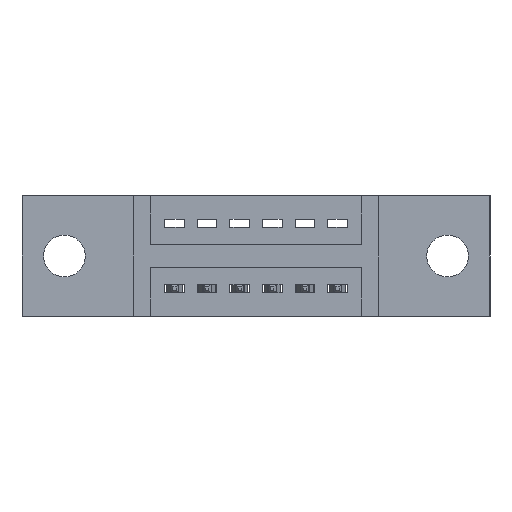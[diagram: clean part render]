
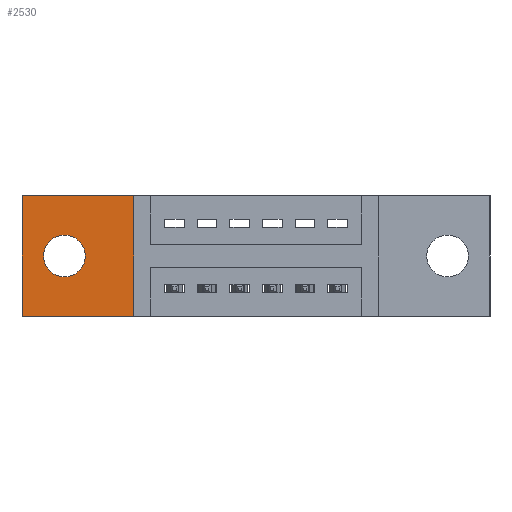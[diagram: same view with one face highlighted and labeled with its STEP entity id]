
A CAD part, front view. The second image highlights one B-rep face of the part: STEP entity #2530.
In plain terms, the highlighted planar face has unit normal (0, -1, 0).
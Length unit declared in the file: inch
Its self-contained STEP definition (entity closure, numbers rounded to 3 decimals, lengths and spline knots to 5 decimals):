
#359 = CARTESIAN_POINT ( 'NONE',  ( 0.3425, 0.11, 0. ) ) ;
#462 = CARTESIAN_POINT ( 'NONE',  ( 0., 0.11, 0. ) ) ;
#1074 = VERTEX_POINT ( 'NONE', #7972 ) ;
#1160 = DIRECTION ( 'NONE',  ( 0., 0., -1. ) ) ;
#1195 = EDGE_CURVE ( 'NONE', #3019, #8788, #3994, .T. ) ;
#1220 = FACE_OUTER_BOUND ( 'NONE', #4221, .T. ) ;
#1246 = CARTESIAN_POINT ( 'NONE',  ( 0., 0.11, 0. ) ) ;
#1267 = EDGE_CURVE ( 'NONE', #8788, #7322, #4454, .T. ) ;
#1342 = AXIS2_PLACEMENT_3D ( 'NONE', #3920, #8228, #3813 ) ;
#1652 = ORIENTED_EDGE ( 'NONE', *, *, #5545, .T. ) ;
#1711 = CARTESIAN_POINT ( 'NONE',  ( 0.3425, 0.11, -0.37 ) ) ;
#1998 = VERTEX_POINT ( 'NONE', #4683 ) ;
#2013 = DIRECTION ( 'NONE',  ( -1., 0., 0. ) ) ;
#2136 = CARTESIAN_POINT ( 'NONE',  ( 0.3425, 0.11, 0. ) ) ;
#2402 = ORIENTED_EDGE ( 'NONE', *, *, #1267, .T. ) ;
#2413 = PLANE ( 'NONE',  #1342 ) ;
#2455 = VECTOR ( 'NONE', #8873, 39.37008 ) ;
#2530 = ADVANCED_FACE ( 'NONE', ( #9464, #1220 ), #2413, .T. ) ;
#2647 = VECTOR ( 'NONE', #2013, 39.37008 ) ;
#2788 = ORIENTED_EDGE ( 'NONE', *, *, #4049, .F. ) ;
#2811 = VERTEX_POINT ( 'NONE', #359 ) ;
#2861 = CARTESIAN_POINT ( 'NONE',  ( 0., 0.11, 0. ) ) ;
#3019 = VERTEX_POINT ( 'NONE', #462 ) ;
#3285 = ORIENTED_EDGE ( 'NONE', *, *, #1195, .T. ) ;
#3395 = CIRCLE ( 'NONE', #6272, 0.064 ) ;
#3813 = DIRECTION ( 'NONE',  ( 0., 0., -1. ) ) ;
#3920 = CARTESIAN_POINT ( 'NONE',  ( 0., 0.11, -0.37 ) ) ;
#3994 = LINE ( 'NONE', #2861, #4461 ) ;
#4049 = EDGE_CURVE ( 'NONE', #1074, #1998, #6425, .T. ) ;
#4217 = DIRECTION ( 'NONE',  ( 0., -1., 0. ) ) ;
#4221 = EDGE_LOOP ( 'NONE', ( #3285, #2402, #6477, #1652 ) ) ;
#4454 = LINE ( 'NONE', #7553, #2455 ) ;
#4461 = VECTOR ( 'NONE', #9439, 39.37008 ) ;
#4683 = CARTESIAN_POINT ( 'NONE',  ( 0.13, 0.11, -0.121 ) ) ;
#4914 = CARTESIAN_POINT ( 'NONE',  ( 0.13, 0.11, -0.185 ) ) ;
#5545 = EDGE_CURVE ( 'NONE', #2811, #3019, #5575, .T. ) ;
#5575 = LINE ( 'NONE', #1246, #2647 ) ;
#5652 = DIRECTION ( 'NONE',  ( 0., -1., 0. ) ) ;
#5697 = VECTOR ( 'NONE', #6621, 39.37008 ) ;
#6240 = AXIS2_PLACEMENT_3D ( 'NONE', #4914, #5652, #1160 ) ;
#6272 = AXIS2_PLACEMENT_3D ( 'NONE', #8012, #4217, #8728 ) ;
#6278 = EDGE_LOOP ( 'NONE', ( #8051, #2788 ) ) ;
#6285 = EDGE_CURVE ( 'NONE', #1998, #1074, #3395, .T. ) ;
#6409 = EDGE_CURVE ( 'NONE', #7322, #2811, #7639, .T. ) ;
#6425 = CIRCLE ( 'NONE', #6240, 0.064 ) ;
#6477 = ORIENTED_EDGE ( 'NONE', *, *, #6409, .T. ) ;
#6621 = DIRECTION ( 'NONE',  ( 0., 0., 1. ) ) ;
#7322 = VERTEX_POINT ( 'NONE', #1711 ) ;
#7553 = CARTESIAN_POINT ( 'NONE',  ( 0., 0.11, -0.37 ) ) ;
#7639 = LINE ( 'NONE', #2136, #5697 ) ;
#7972 = CARTESIAN_POINT ( 'NONE',  ( 0.13, 0.11, -0.249 ) ) ;
#8012 = CARTESIAN_POINT ( 'NONE',  ( 0.13, 0.11, -0.185 ) ) ;
#8051 = ORIENTED_EDGE ( 'NONE', *, *, #6285, .F. ) ;
#8228 = DIRECTION ( 'NONE',  ( 0., -1., 0. ) ) ;
#8728 = DIRECTION ( 'NONE',  ( 0., 0., -1. ) ) ;
#8788 = VERTEX_POINT ( 'NONE', #9242 ) ;
#8873 = DIRECTION ( 'NONE',  ( 1., 0., 0. ) ) ;
#9242 = CARTESIAN_POINT ( 'NONE',  ( 0., 0.11, -0.37 ) ) ;
#9439 = DIRECTION ( 'NONE',  ( 0., 0., -1. ) ) ;
#9464 = FACE_BOUND ( 'NONE', #6278, .T. ) ;
